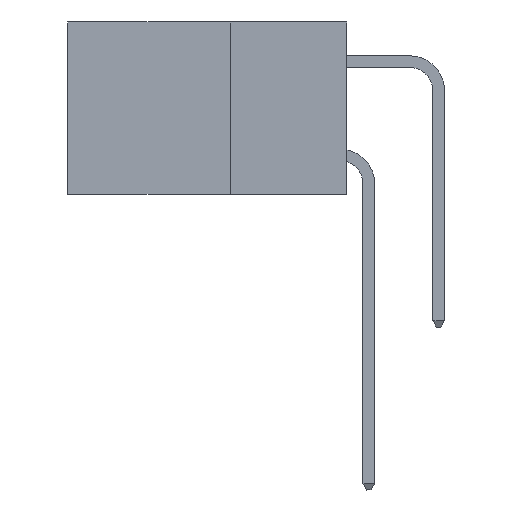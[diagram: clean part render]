
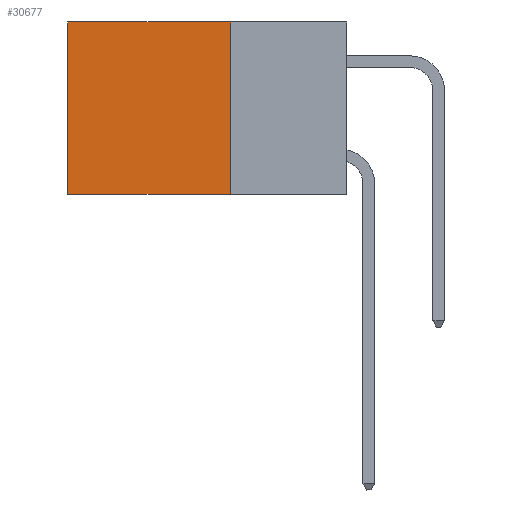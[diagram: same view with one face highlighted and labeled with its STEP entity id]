
A CAD part, left-side view. The second image highlights one B-rep face of the part: STEP entity #30677.
In plain terms, the highlighted planar face has unit normal (-1, 0, 0).
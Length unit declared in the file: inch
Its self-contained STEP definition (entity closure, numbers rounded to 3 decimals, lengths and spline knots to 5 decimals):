
#1138 = VERTEX_POINT ( 'NONE', #4199 ) ;
#1608 = CARTESIAN_POINT ( 'NONE',  ( 0.2875, 0.25, 0. ) ) ;
#2144 = EDGE_CURVE ( 'NONE', #27763, #10191, #20299, .T. ) ;
#3112 = CARTESIAN_POINT ( 'NONE',  ( 0.2875, 0.6, 0. ) ) ;
#3189 = DIRECTION ( 'NONE',  ( 1., 0., 0. ) ) ;
#4199 = CARTESIAN_POINT ( 'NONE',  ( 0.2875, 0.25, -0.37 ) ) ;
#10191 = VERTEX_POINT ( 'NONE', #26214 ) ;
#11119 = DIRECTION ( 'NONE',  ( 0., 0., -1. ) ) ;
#13008 = VECTOR ( 'NONE', #19368, 39.37008 ) ;
#13761 = CARTESIAN_POINT ( 'NONE',  ( 0.2875, 0.25, 0. ) ) ;
#15033 = FACE_OUTER_BOUND ( 'NONE', #20195, .T. ) ;
#15728 = DIRECTION ( 'NONE',  ( 0., 0., -1. ) ) ;
#18036 = CARTESIAN_POINT ( 'NONE',  ( 0.2875, 0.6, 0. ) ) ;
#18285 = CARTESIAN_POINT ( 'NONE',  ( 0.2875, 0.25, 0. ) ) ;
#19368 = DIRECTION ( 'NONE',  ( 0., 1., 0. ) ) ;
#19673 = EDGE_CURVE ( 'NONE', #30799, #1138, #23433, .T. ) ;
#19730 = LINE ( 'NONE', #32397, #13008 ) ;
#19735 = ORIENTED_EDGE ( 'NONE', *, *, #19673, .F. ) ;
#19816 = DIRECTION ( 'NONE',  ( 0., 1., 0. ) ) ;
#20195 = EDGE_LOOP ( 'NONE', ( #25100, #20909, #19735, #31260 ) ) ;
#20299 = LINE ( 'NONE', #18036, #21451 ) ;
#20376 = AXIS2_PLACEMENT_3D ( 'NONE', #18285, #3189, #11119 ) ;
#20909 = ORIENTED_EDGE ( 'NONE', *, *, #31494, .F. ) ;
#21206 = DIRECTION ( 'NONE',  ( 0., 0., -1. ) ) ;
#21290 = PLANE ( 'NONE',  #20376 ) ;
#21451 = VECTOR ( 'NONE', #15728, 39.37008 ) ;
#21473 = VECTOR ( 'NONE', #19816, 39.37008 ) ;
#21482 = VECTOR ( 'NONE', #21206, 39.37008 ) ;
#23433 = LINE ( 'NONE', #28884, #21482 ) ;
#25100 = ORIENTED_EDGE ( 'NONE', *, *, #2144, .T. ) ;
#25194 = EDGE_CURVE ( 'NONE', #30799, #27763, #28520, .T. ) ;
#26214 = CARTESIAN_POINT ( 'NONE',  ( 0.2875, 0.6, -0.37 ) ) ;
#27763 = VERTEX_POINT ( 'NONE', #3112 ) ;
#28520 = LINE ( 'NONE', #1608, #21473 ) ;
#28884 = CARTESIAN_POINT ( 'NONE',  ( 0.2875, 0.25, 0. ) ) ;
#30677 = ADVANCED_FACE ( 'NONE', ( #15033 ), #21290, .F. ) ;
#30799 = VERTEX_POINT ( 'NONE', #13761 ) ;
#31260 = ORIENTED_EDGE ( 'NONE', *, *, #25194, .T. ) ;
#31494 = EDGE_CURVE ( 'NONE', #1138, #10191, #19730, .T. ) ;
#32397 = CARTESIAN_POINT ( 'NONE',  ( 0.2875, 0.25, -0.37 ) ) ;
